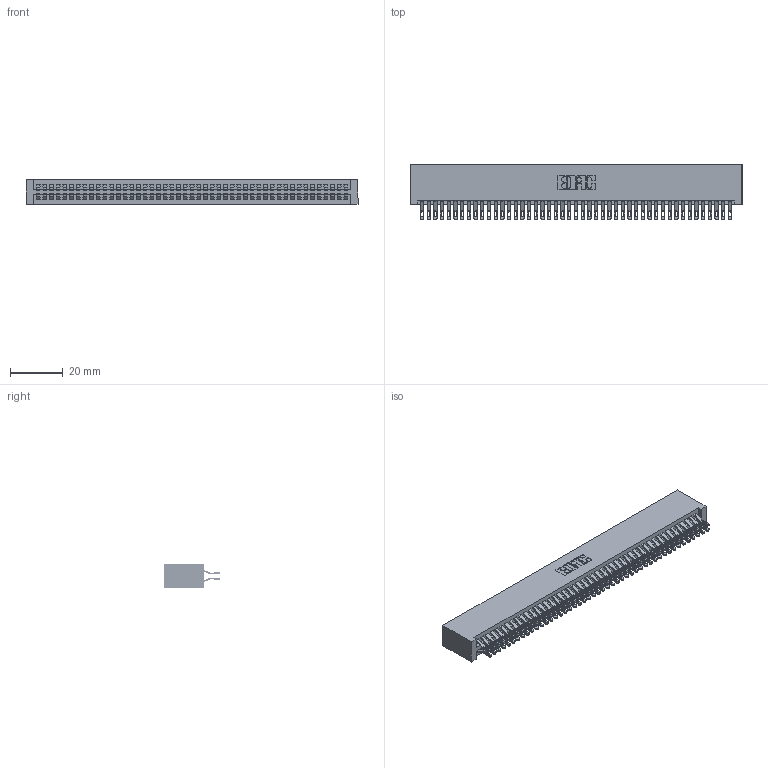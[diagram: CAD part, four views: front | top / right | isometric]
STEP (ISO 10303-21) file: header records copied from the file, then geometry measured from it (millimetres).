
FILE_DESCRIPTION (( 'STEP AP203' ), '1' );
FILE_NAME ('395-094-555-201.STEP', '2018-11-29T13:27:43', ( '' ), ( '' ), 'SwSTEP 2.0', 'SolidWorks 2016', '' );
FILE_SCHEMA (( 'CONFIG_CONTROL_DESIGN' ));
Length unit declared in the file: inch
Products named in the file (3): 345 Part_No Mounting Lugs; 345-292-001_555 Tail; 395-094-555-201
Assembly tree (95 placements, depth 2):
  395-094-555-201
    345 Part_No Mounting Lugs
    345-292-001_555 Tail  x94
Bounding box: 125.98 x 21.13 x 9.4 mm (x, y, z)
Volume: 13173.2 mm3; surface area: 20820.6 mm2
Topology: 95 solids, 95 shells, 5382 faces, 16955 edges, 11302 vertices
Faces by surface type: plane 2990, cylinder 2392
Entity records: 36253 total; most frequent: CARTESIAN_POINT 6106, ORIENTED_EDGE 6010, DIRECTION 5341, EDGE_CURVE 3005, LINE 2673, VECTOR 2673, VERTEX_POINT 2002, AXIS2_PLACEMENT_3D 1334
